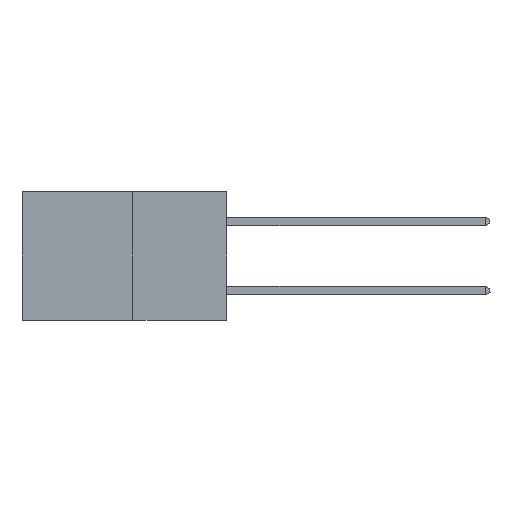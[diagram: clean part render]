
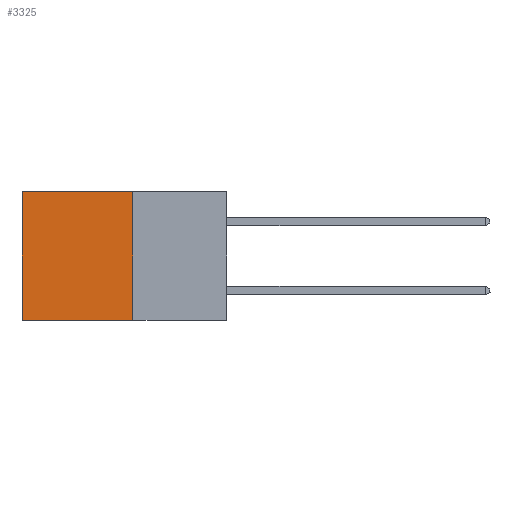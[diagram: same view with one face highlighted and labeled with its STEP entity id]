
A CAD part, left-side view. The second image highlights one B-rep face of the part: STEP entity #3325.
In plain terms, the highlighted planar face has unit normal (-1, 0, 0).
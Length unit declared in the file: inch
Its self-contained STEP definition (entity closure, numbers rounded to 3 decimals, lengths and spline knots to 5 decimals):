
#111 = CARTESIAN_POINT ( 'NONE',  ( 0.277, 0.27, -0.37 ) ) ;
#630 = EDGE_CURVE ( 'NONE', #3572, #8779, #6922, .T. ) ;
#1025 = EDGE_CURVE ( 'NONE', #5234, #3572, #4721, .T. ) ;
#1245 = CARTESIAN_POINT ( 'NONE',  ( 0.277, 0.27, 0. ) ) ;
#1322 = DIRECTION ( 'NONE',  ( 0., 1., 0. ) ) ;
#1417 = VECTOR ( 'NONE', #1322, 39.37008 ) ;
#1951 = CARTESIAN_POINT ( 'NONE',  ( 0.277, 0.59, 0. ) ) ;
#2002 = AXIS2_PLACEMENT_3D ( 'NONE', #6847, #6358, #6205 ) ;
#2227 = CARTESIAN_POINT ( 'NONE',  ( 0.277, 0.27, 0. ) ) ;
#2534 = VECTOR ( 'NONE', #2631, 39.37008 ) ;
#2631 = DIRECTION ( 'NONE',  ( 0., 1., 0. ) ) ;
#2700 = DIRECTION ( 'NONE',  ( 0., 0., -1. ) ) ;
#2843 = EDGE_LOOP ( 'NONE', ( #5078, #6594, #4670, #5797 ) ) ;
#3325 = ADVANCED_FACE ( 'NONE', ( #5838 ), #6978, .F. ) ;
#3572 = VERTEX_POINT ( 'NONE', #8786 ) ;
#4307 = CARTESIAN_POINT ( 'NONE',  ( 0.277, 0.27, -0.37 ) ) ;
#4670 = ORIENTED_EDGE ( 'NONE', *, *, #1025, .F. ) ;
#4714 = CARTESIAN_POINT ( 'NONE',  ( 0.277, 0.59, -0.37 ) ) ;
#4721 = LINE ( 'NONE', #111, #7998 ) ;
#4767 = DIRECTION ( 'NONE',  ( 0., 0., -1. ) ) ;
#5078 = ORIENTED_EDGE ( 'NONE', *, *, #7002, .T. ) ;
#5234 = VERTEX_POINT ( 'NONE', #2227 ) ;
#5280 = VERTEX_POINT ( 'NONE', #1951 ) ;
#5470 = EDGE_CURVE ( 'NONE', #5234, #5280, #5701, .T. ) ;
#5701 = LINE ( 'NONE', #1245, #1417 ) ;
#5797 = ORIENTED_EDGE ( 'NONE', *, *, #5470, .T. ) ;
#5838 = FACE_OUTER_BOUND ( 'NONE', #2843, .T. ) ;
#6205 = DIRECTION ( 'NONE',  ( 0., 0., -1. ) ) ;
#6358 = DIRECTION ( 'NONE',  ( 1., 0., 0. ) ) ;
#6365 = VECTOR ( 'NONE', #4767, 39.37008 ) ;
#6594 = ORIENTED_EDGE ( 'NONE', *, *, #630, .F. ) ;
#6847 = CARTESIAN_POINT ( 'NONE',  ( 0.277, 0.27, -0.37 ) ) ;
#6882 = CARTESIAN_POINT ( 'NONE',  ( 0.277, 0.59, -0.37 ) ) ;
#6922 = LINE ( 'NONE', #4307, #2534 ) ;
#6978 = PLANE ( 'NONE',  #2002 ) ;
#7002 = EDGE_CURVE ( 'NONE', #5280, #8779, #8922, .T. ) ;
#7998 = VECTOR ( 'NONE', #2700, 39.37008 ) ;
#8779 = VERTEX_POINT ( 'NONE', #6882 ) ;
#8786 = CARTESIAN_POINT ( 'NONE',  ( 0.277, 0.27, -0.37 ) ) ;
#8922 = LINE ( 'NONE', #4714, #6365 ) ;
